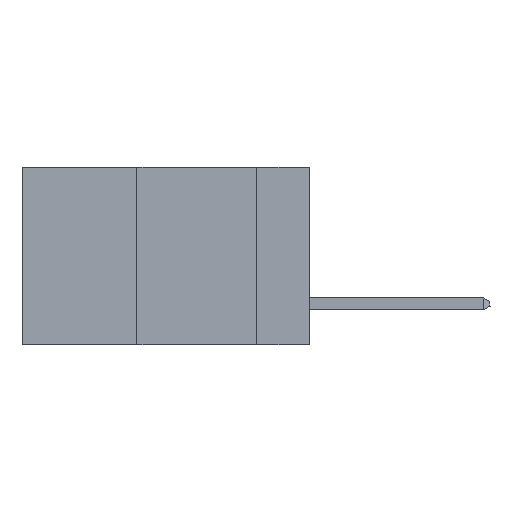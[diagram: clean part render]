
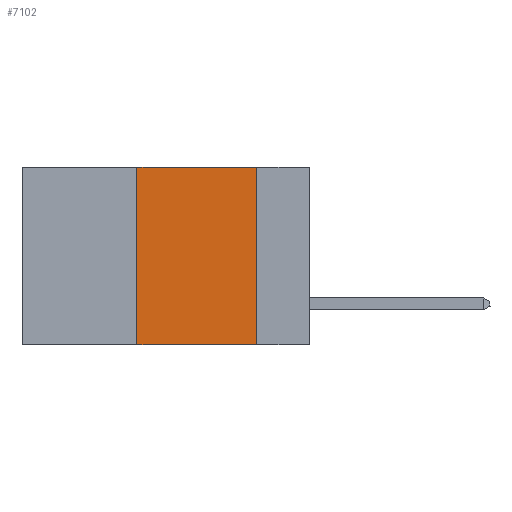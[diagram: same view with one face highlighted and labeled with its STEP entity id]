
A CAD part, left-side view. The second image highlights one B-rep face of the part: STEP entity #7102.
In plain terms, the highlighted planar face has unit normal (-1, 0, 0).
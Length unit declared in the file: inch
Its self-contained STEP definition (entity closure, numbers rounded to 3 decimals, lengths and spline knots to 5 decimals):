
#1157 = CARTESIAN_POINT ( 'NONE',  ( 0., 0.6, -0.37 ) ) ;
#1346 = VERTEX_POINT ( 'NONE', #7495 ) ;
#2932 = LINE ( 'NONE', #1157, #3788 ) ;
#3788 = VECTOR ( 'NONE', #30790, 39.37008 ) ;
#4450 = VERTEX_POINT ( 'NONE', #16440 ) ;
#4468 = EDGE_CURVE ( 'NONE', #21499, #4450, #23162, .T. ) ;
#5325 = VECTOR ( 'NONE', #10076, 39.37008 ) ;
#5898 = EDGE_CURVE ( 'NONE', #1346, #24948, #2932, .T. ) ;
#6468 = DIRECTION ( 'NONE',  ( 0., 0., -1. ) ) ;
#7102 = ADVANCED_FACE ( 'NONE', ( #29361 ), #12101, .F. ) ;
#7495 = CARTESIAN_POINT ( 'NONE',  ( 0., 0.36, -0.37 ) ) ;
#10076 = DIRECTION ( 'NONE',  ( 0., 0., 1. ) ) ;
#11170 = VECTOR ( 'NONE', #29931, 39.37008 ) ;
#12101 = PLANE ( 'NONE',  #32151 ) ;
#12691 = DIRECTION ( 'NONE',  ( 0., 0., -1. ) ) ;
#16159 = LINE ( 'NONE', #29031, #22175 ) ;
#16440 = CARTESIAN_POINT ( 'NONE',  ( 0., 0.11, 0. ) ) ;
#17254 = DIRECTION ( 'NONE',  ( 1., 0., 0. ) ) ;
#18596 = CARTESIAN_POINT ( 'NONE',  ( 0., 0.36, 0. ) ) ;
#21065 = CARTESIAN_POINT ( 'NONE',  ( 0., 0.36, 0. ) ) ;
#21270 = ORIENTED_EDGE ( 'NONE', *, *, #23146, .F. ) ;
#21499 = VERTEX_POINT ( 'NONE', #18596 ) ;
#22175 = VECTOR ( 'NONE', #12691, 39.37008 ) ;
#22767 = CARTESIAN_POINT ( 'NONE',  ( 0., 0.11, -0.37 ) ) ;
#23146 = EDGE_CURVE ( 'NONE', #1346, #21499, #26715, .T. ) ;
#23162 = LINE ( 'NONE', #27426, #11170 ) ;
#23574 = EDGE_LOOP ( 'NONE', ( #31591, #29682, #21270, #28639 ) ) ;
#24948 = VERTEX_POINT ( 'NONE', #22767 ) ;
#26715 = LINE ( 'NONE', #21065, #5325 ) ;
#27426 = CARTESIAN_POINT ( 'NONE',  ( 0., 0.6, 0. ) ) ;
#28639 = ORIENTED_EDGE ( 'NONE', *, *, #5898, .T. ) ;
#29031 = CARTESIAN_POINT ( 'NONE',  ( 0., 0.11, 0. ) ) ;
#29361 = FACE_OUTER_BOUND ( 'NONE', #23574, .T. ) ;
#29682 = ORIENTED_EDGE ( 'NONE', *, *, #4468, .F. ) ;
#29931 = DIRECTION ( 'NONE',  ( 0., -1., 0. ) ) ;
#30790 = DIRECTION ( 'NONE',  ( 0., -1., 0. ) ) ;
#31189 = CARTESIAN_POINT ( 'NONE',  ( 0., 0.6, 0. ) ) ;
#31591 = ORIENTED_EDGE ( 'NONE', *, *, #33299, .F. ) ;
#32151 = AXIS2_PLACEMENT_3D ( 'NONE', #31189, #17254, #6468 ) ;
#33299 = EDGE_CURVE ( 'NONE', #4450, #24948, #16159, .T. ) ;
